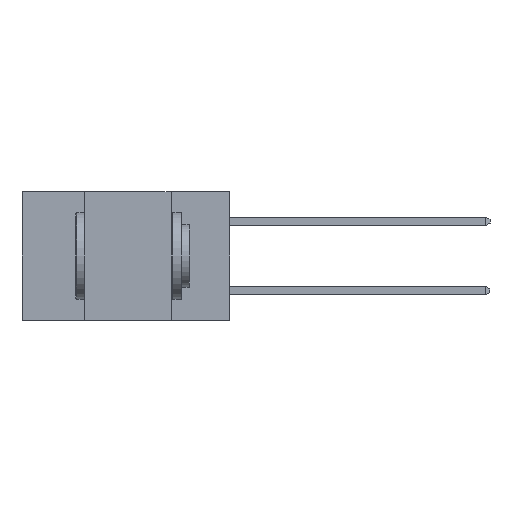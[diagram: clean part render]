
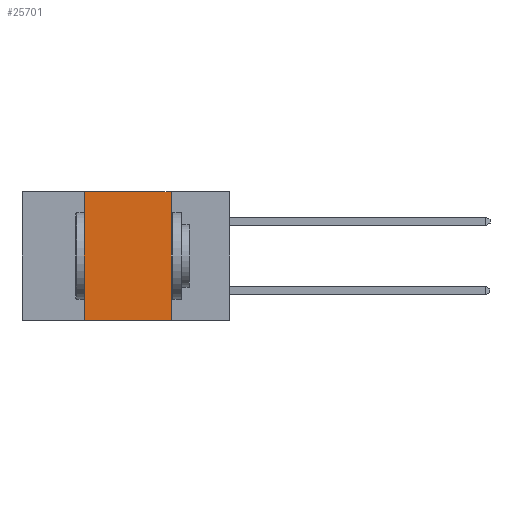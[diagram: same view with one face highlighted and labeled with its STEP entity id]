
A CAD part, left-side view. The second image highlights one B-rep face of the part: STEP entity #25701.
In plain terms, the highlighted planar face has unit normal (-1, 0, 0).
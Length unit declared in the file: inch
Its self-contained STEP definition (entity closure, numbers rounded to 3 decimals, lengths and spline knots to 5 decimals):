
#1575 = EDGE_CURVE ( 'NONE', #15347, #20363, #7980, .T. ) ;
#1580 = CARTESIAN_POINT ( 'NONE',  ( 0., 0.42, 0. ) ) ;
#1748 = CARTESIAN_POINT ( 'NONE',  ( 0., 0.17, 0. ) ) ;
#3166 = EDGE_LOOP ( 'NONE', ( #21738, #11152, #5978, #5850 ) ) ;
#3756 = LINE ( 'NONE', #25530, #19807 ) ;
#4612 = CARTESIAN_POINT ( 'NONE',  ( 0., 0.6, 0. ) ) ;
#5202 = LINE ( 'NONE', #25248, #21218 ) ;
#5850 = ORIENTED_EDGE ( 'NONE', *, *, #20744, .T. ) ;
#5978 = ORIENTED_EDGE ( 'NONE', *, *, #6479, .F. ) ;
#6479 = EDGE_CURVE ( 'NONE', #8796, #15347, #15771, .T. ) ;
#6813 = DIRECTION ( 'NONE',  ( 0., 0., -1. ) ) ;
#7969 = CARTESIAN_POINT ( 'NONE',  ( 0., 0.17, -0.37 ) ) ;
#7980 = LINE ( 'NONE', #27443, #14492 ) ;
#8796 = VERTEX_POINT ( 'NONE', #21281 ) ;
#9408 = EDGE_CURVE ( 'NONE', #20363, #11038, #3756, .T. ) ;
#9963 = VECTOR ( 'NONE', #25575, 39.37008 ) ;
#11038 = VERTEX_POINT ( 'NONE', #7969 ) ;
#11152 = ORIENTED_EDGE ( 'NONE', *, *, #1575, .F. ) ;
#14426 = DIRECTION ( 'NONE',  ( 0., -1., 0. ) ) ;
#14492 = VECTOR ( 'NONE', #14426, 39.37008 ) ;
#15347 = VERTEX_POINT ( 'NONE', #17242 ) ;
#15771 = LINE ( 'NONE', #1580, #9963 ) ;
#17242 = CARTESIAN_POINT ( 'NONE',  ( 0., 0.42, 0. ) ) ;
#17670 = PLANE ( 'NONE',  #26519 ) ;
#19807 = VECTOR ( 'NONE', #27730, 39.37008 ) ;
#19882 = DIRECTION ( 'NONE',  ( 1., 0., 0. ) ) ;
#20363 = VERTEX_POINT ( 'NONE', #1748 ) ;
#20744 = EDGE_CURVE ( 'NONE', #8796, #11038, #5202, .T. ) ;
#21218 = VECTOR ( 'NONE', #25147, 39.37008 ) ;
#21281 = CARTESIAN_POINT ( 'NONE',  ( 0., 0.42, -0.37 ) ) ;
#21738 = ORIENTED_EDGE ( 'NONE', *, *, #9408, .F. ) ;
#23434 = FACE_OUTER_BOUND ( 'NONE', #3166, .T. ) ;
#25147 = DIRECTION ( 'NONE',  ( 0., -1., 0. ) ) ;
#25248 = CARTESIAN_POINT ( 'NONE',  ( 0., 0.6, -0.37 ) ) ;
#25530 = CARTESIAN_POINT ( 'NONE',  ( 0., 0.17, 0. ) ) ;
#25575 = DIRECTION ( 'NONE',  ( 0., 0., 1. ) ) ;
#25701 = ADVANCED_FACE ( 'NONE', ( #23434 ), #17670, .F. ) ;
#26519 = AXIS2_PLACEMENT_3D ( 'NONE', #4612, #19882, #6813 ) ;
#27443 = CARTESIAN_POINT ( 'NONE',  ( 0., 0.6, 0. ) ) ;
#27730 = DIRECTION ( 'NONE',  ( 0., 0., -1. ) ) ;
